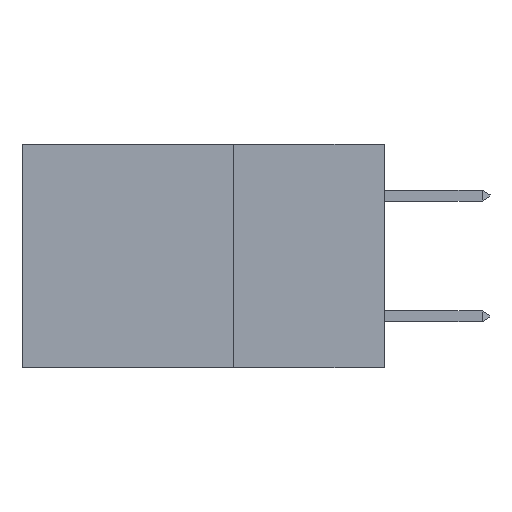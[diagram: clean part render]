
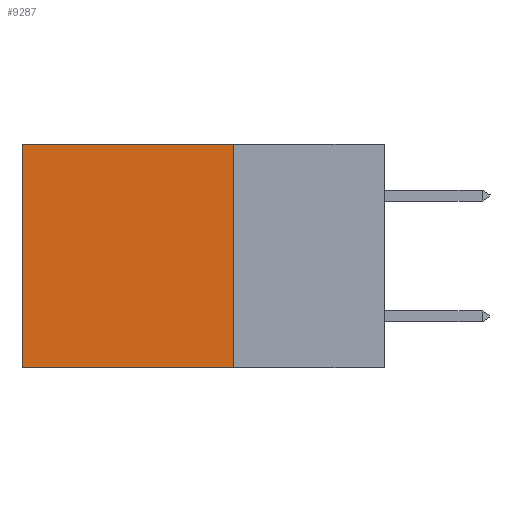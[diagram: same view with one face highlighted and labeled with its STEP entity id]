
A CAD part, left-side view. The second image highlights one B-rep face of the part: STEP entity #9287.
In plain terms, the highlighted planar face has unit normal (-1, 0, 0).
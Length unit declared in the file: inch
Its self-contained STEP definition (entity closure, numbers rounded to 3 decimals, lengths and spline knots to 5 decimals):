
#1264 = CARTESIAN_POINT ( 'NONE',  ( 0.2875, 0.6, 0. ) ) ;
#3284 = CARTESIAN_POINT ( 'NONE',  ( 0.2875, 0.25, 0. ) ) ;
#3289 = CARTESIAN_POINT ( 'NONE',  ( 0.2875, 0.25, 0. ) ) ;
#5434 = DIRECTION ( 'NONE',  ( 0., 0., -1. ) ) ;
#6001 = CARTESIAN_POINT ( 'NONE',  ( 0.2875, 0.6, -0.37 ) ) ;
#6334 = VERTEX_POINT ( 'NONE', #6001 ) ;
#9287 = ADVANCED_FACE ( 'NONE', ( #9661 ), #38673, .F. ) ;
#9661 = FACE_OUTER_BOUND ( 'NONE', #27871, .T. ) ;
#10503 = LINE ( 'NONE', #3284, #30534 ) ;
#11630 = CARTESIAN_POINT ( 'NONE',  ( 0.2875, 0.25, 0. ) ) ;
#11791 = VECTOR ( 'NONE', #38092, 39.37008 ) ;
#12614 = VERTEX_POINT ( 'NONE', #37585 ) ;
#13189 = DIRECTION ( 'NONE',  ( 0., 0., -1. ) ) ;
#13905 = CARTESIAN_POINT ( 'NONE',  ( 0.2875, 0.25, -0.37 ) ) ;
#14494 = VECTOR ( 'NONE', #5434, 39.37008 ) ;
#14657 = VERTEX_POINT ( 'NONE', #3289 ) ;
#15869 = LINE ( 'NONE', #11630, #14494 ) ;
#18178 = LINE ( 'NONE', #1264, #24356 ) ;
#18699 = ORIENTED_EDGE ( 'NONE', *, *, #24208, .T. ) ;
#20486 = DIRECTION ( 'NONE',  ( 1., 0., 0. ) ) ;
#22677 = EDGE_CURVE ( 'NONE', #14657, #23751, #15869, .T. ) ;
#22844 = CARTESIAN_POINT ( 'NONE',  ( 0.2875, 0.25, -0.37 ) ) ;
#23751 = VERTEX_POINT ( 'NONE', #13905 ) ;
#24208 = EDGE_CURVE ( 'NONE', #14657, #12614, #10503, .T. ) ;
#24312 = EDGE_CURVE ( 'NONE', #12614, #6334, #18178, .T. ) ;
#24356 = VECTOR ( 'NONE', #13189, 39.37008 ) ;
#25820 = ORIENTED_EDGE ( 'NONE', *, *, #28945, .F. ) ;
#27012 = CARTESIAN_POINT ( 'NONE',  ( 0.2875, 0.25, 0. ) ) ;
#27871 = EDGE_LOOP ( 'NONE', ( #37454, #25820, #31695, #18699 ) ) ;
#28945 = EDGE_CURVE ( 'NONE', #23751, #6334, #33217, .T. ) ;
#30534 = VECTOR ( 'NONE', #34082, 39.37008 ) ;
#31695 = ORIENTED_EDGE ( 'NONE', *, *, #22677, .F. ) ;
#33073 = AXIS2_PLACEMENT_3D ( 'NONE', #27012, #20486, #35925 ) ;
#33217 = LINE ( 'NONE', #22844, #11791 ) ;
#34082 = DIRECTION ( 'NONE',  ( 0., 1., 0. ) ) ;
#35925 = DIRECTION ( 'NONE',  ( 0., 0., -1. ) ) ;
#37454 = ORIENTED_EDGE ( 'NONE', *, *, #24312, .T. ) ;
#37585 = CARTESIAN_POINT ( 'NONE',  ( 0.2875, 0.6, 0. ) ) ;
#38092 = DIRECTION ( 'NONE',  ( 0., 1., 0. ) ) ;
#38673 = PLANE ( 'NONE',  #33073 ) ;
